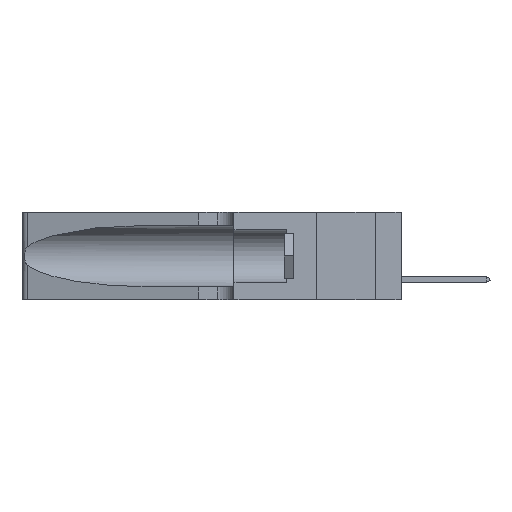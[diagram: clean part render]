
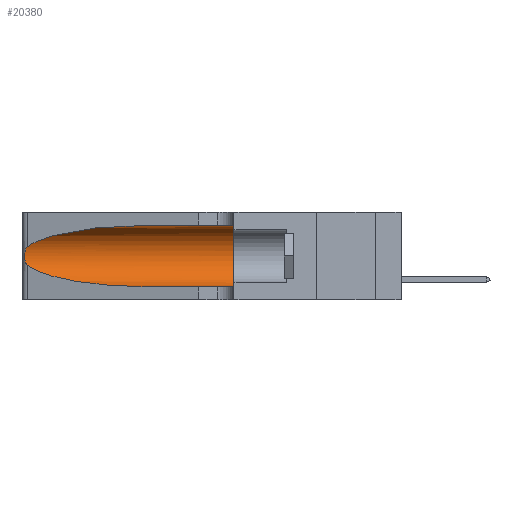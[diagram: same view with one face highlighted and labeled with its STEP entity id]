
A CAD part, left-side view. The second image highlights one B-rep face of the part: STEP entity #20380.
In plain terms, the highlighted cylindrical face has radius 3.308 mm (diameter 6.617 mm), a partial arc.
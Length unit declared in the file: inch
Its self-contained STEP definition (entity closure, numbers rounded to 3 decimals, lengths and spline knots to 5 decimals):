
#326 = DIRECTION ( 'NONE',  ( 0., -1., 0. ) ) ;
#334 = ORIENTED_EDGE ( 'NONE', *, *, #17800, .T. ) ;
#419 = CARTESIAN_POINT ( 'NONE',  ( 0.26075, 1.23896, 0.19203 ) ) ;
#565 = CARTESIAN_POINT ( 'NONE',  ( 0.25639, 1.23186, 0.15144 ) ) ;
#1306 = CARTESIAN_POINT ( 'NONE',  ( 0.1305, 0.72297, 0.31525 ) ) ;
#1899 = EDGE_CURVE ( 'NONE', #34600, #44005, #41980, .T. ) ;
#3852 = EDGE_LOOP ( 'NONE', ( #35251, #334, #13677, #14131, #32167, #5643 ) ) ;
#4461 = DIRECTION ( 'NONE',  ( 0., -1., 0. ) ) ;
#4888 = DIRECTION ( 'NONE',  ( 0., 0., 1. ) ) ;
#4912 = EDGE_CURVE ( 'NONE', #15564, #35276, #20714, .T. ) ;
#5643 = ORIENTED_EDGE ( 'NONE', *, *, #4912, .F. ) ;
#5719 = CARTESIAN_POINT ( 'NONE',  ( 0.25487, 1.22718, 0.14631 ) ) ;
#7295 = CARTESIAN_POINT ( 'NONE',  ( 0.18966, 0.96281, 0.05475 ) ) ;
#7487 = EDGE_CURVE ( 'NONE', #35276, #23246, #8809, .T. ) ;
#8809 = CIRCLE ( 'NONE', #9973, 0.13025 ) ;
#9056 = DIRECTION ( 'NONE',  ( 0., 1., 0. ) ) ;
#9284 = FACE_OUTER_BOUND ( 'NONE', #3852, .T. ) ;
#9973 = AXIS2_PLACEMENT_3D ( 'NONE', #25708, #9056, #4888 ) ;
#11184 = CARTESIAN_POINT ( 'NONE',  ( 0.1305, 0.35, 0.05475 ) ) ;
#12354 = DIRECTION ( 'NONE',  ( 0., 0., -1. ) ) ;
#12380 = LINE ( 'NONE', #15000, #36065 ) ;
#13560 = VECTOR ( 'NONE', #42159, 39.37008 ) ;
#13677 = ORIENTED_EDGE ( 'NONE', *, *, #1899, .T. ) ;
#14131 = ORIENTED_EDGE ( 'NONE', *, *, #34795, .T. ) ;
#15000 = CARTESIAN_POINT ( 'NONE',  ( 0.1305, 1.61858, 0.05475 ) ) ;
#15098 = CARTESIAN_POINT ( 'NONE',  ( 0.25789, 1.23486, 0.15765 ) ) ;
#15564 = VERTEX_POINT ( 'NONE', #1306 ) ;
#16666 = CARTESIAN_POINT ( 'NONE',  ( 0.18966, 0.96281, 0.31525 ) ) ;
#16818 = CARTESIAN_POINT ( 'NONE',  ( 0.2373, 1.15595, 0.28018 ) ) ;
#16926 = CARTESIAN_POINT ( 'NONE',  ( 0.25487, 1.22718, 0.14631 ) ) ;
#16971 = CARTESIAN_POINT ( 'NONE',  ( 0.1305, 0.72297, 0.31525 ) ) ;
#17493 = CARTESIAN_POINT ( 'NONE',  ( 0.1305, 1.61858, 0.31525 ) ) ;
#17800 = EDGE_CURVE ( 'NONE', #25145, #34600, #22196, .T. ) ;
#18459 = CARTESIAN_POINT ( 'NONE',  ( 0.26075, 1.23896, 0.178 ) ) ;
#19373 =( BOUNDED_CURVE ( )  B_SPLINE_CURVE ( 3, ( #16971, #16666, #16818, #30744 ),
 .UNSPECIFIED., .F., .T. ) 
 B_SPLINE_CURVE_WITH_KNOTS ( ( 4, 4 ),
 ( 1.5708, 2.84003 ),
 .UNSPECIFIED. ) 
 CURVE ( )  GEOMETRIC_REPRESENTATION_ITEM ( )  RATIONAL_B_SPLINE_CURVE ( ( 1., 0.87, 0.87, 1. ) ) 
 REPRESENTATION_ITEM ( '' )  );
#20380 = ADVANCED_FACE ( 'NONE', ( #9284 ), #38526, .F. ) ;
#20714 = LINE ( 'NONE', #17493, #13560 ) ;
#21237 = CARTESIAN_POINT ( 'NONE',  ( 0.2373, 1.15595, 0.08982 ) ) ;
#21725 = CARTESIAN_POINT ( 'NONE',  ( 0.26017, 1.23833, 0.17102 ) ) ;
#22196 = B_SPLINE_CURVE_WITH_KNOTS ( 'NONE', 3,
 ( #32098, #35632, #42966, #28995, #39277, #39599, #419, #18459, #21725, #29156, #15098, #565, #39764, #25264 ),
 .UNSPECIFIED., .F., .F.,
 ( 4, 2, 2, 2, 2, 2, 4 ),
 ( 0., 0.00027, 0.00053, 0.00107, 0.0016, 0.00187, 0.00214 ),
 .UNSPECIFIED. ) ;
#23002 = AXIS2_PLACEMENT_3D ( 'NONE', #39479, #4461, #12354 ) ;
#23246 = VERTEX_POINT ( 'NONE', #11184 ) ;
#25145 = VERTEX_POINT ( 'NONE', #25202 ) ;
#25202 = CARTESIAN_POINT ( 'NONE',  ( 0.25487, 1.22718, 0.22369 ) ) ;
#25264 = CARTESIAN_POINT ( 'NONE',  ( 0.25487, 1.22718, 0.14631 ) ) ;
#25708 = CARTESIAN_POINT ( 'NONE',  ( 0.1305, 0.35, 0.185 ) ) ;
#28995 = CARTESIAN_POINT ( 'NONE',  ( 0.25787, 1.23484, 0.2124 ) ) ;
#29156 = CARTESIAN_POINT ( 'NONE',  ( 0.25856, 1.23593, 0.16098 ) ) ;
#30744 = CARTESIAN_POINT ( 'NONE',  ( 0.25487, 1.22718, 0.22369 ) ) ;
#32038 = CARTESIAN_POINT ( 'NONE',  ( 0.1305, 0.72297, 0.05475 ) ) ;
#32098 = CARTESIAN_POINT ( 'NONE',  ( 0.25487, 1.22718, 0.22369 ) ) ;
#32167 = ORIENTED_EDGE ( 'NONE', *, *, #7487, .F. ) ;
#33916 = CARTESIAN_POINT ( 'NONE',  ( 0.1305, 0.72297, 0.05475 ) ) ;
#34600 = VERTEX_POINT ( 'NONE', #5719 ) ;
#34795 = EDGE_CURVE ( 'NONE', #44005, #23246, #12380, .T. ) ;
#35251 = ORIENTED_EDGE ( 'NONE', *, *, #37351, .T. ) ;
#35276 = VERTEX_POINT ( 'NONE', #39162 ) ;
#35632 = CARTESIAN_POINT ( 'NONE',  ( 0.25555, 1.22994, 0.2215 ) ) ;
#36065 = VECTOR ( 'NONE', #326, 39.37008 ) ;
#37351 = EDGE_CURVE ( 'NONE', #15564, #25145, #19373, .T. ) ;
#38526 = CYLINDRICAL_SURFACE ( 'NONE', #23002, 0.13025 ) ;
#39162 = CARTESIAN_POINT ( 'NONE',  ( 0.1305, 0.35, 0.31525 ) ) ;
#39277 = CARTESIAN_POINT ( 'NONE',  ( 0.25854, 1.2359, 0.20912 ) ) ;
#39479 = CARTESIAN_POINT ( 'NONE',  ( 0.1305, 1.61858, 0.185 ) ) ;
#39599 = CARTESIAN_POINT ( 'NONE',  ( 0.26018, 1.23835, 0.19895 ) ) ;
#39764 = CARTESIAN_POINT ( 'NONE',  ( 0.25555, 1.22993, 0.14849 ) ) ;
#41980 =( BOUNDED_CURVE ( )  B_SPLINE_CURVE ( 3, ( #16926, #21237, #7295, #32038 ),
 .UNSPECIFIED., .F., .F. ) 
 B_SPLINE_CURVE_WITH_KNOTS ( ( 4, 4 ),
 ( 3.44316, 4.71239 ),
 .UNSPECIFIED. ) 
 CURVE ( )  GEOMETRIC_REPRESENTATION_ITEM ( )  RATIONAL_B_SPLINE_CURVE ( ( 1., 0.87, 0.87, 1. ) ) 
 REPRESENTATION_ITEM ( '' )  );
#42159 = DIRECTION ( 'NONE',  ( 0., -1., 0. ) ) ;
#42966 = CARTESIAN_POINT ( 'NONE',  ( 0.25639, 1.23184, 0.21858 ) ) ;
#44005 = VERTEX_POINT ( 'NONE', #33916 ) ;
